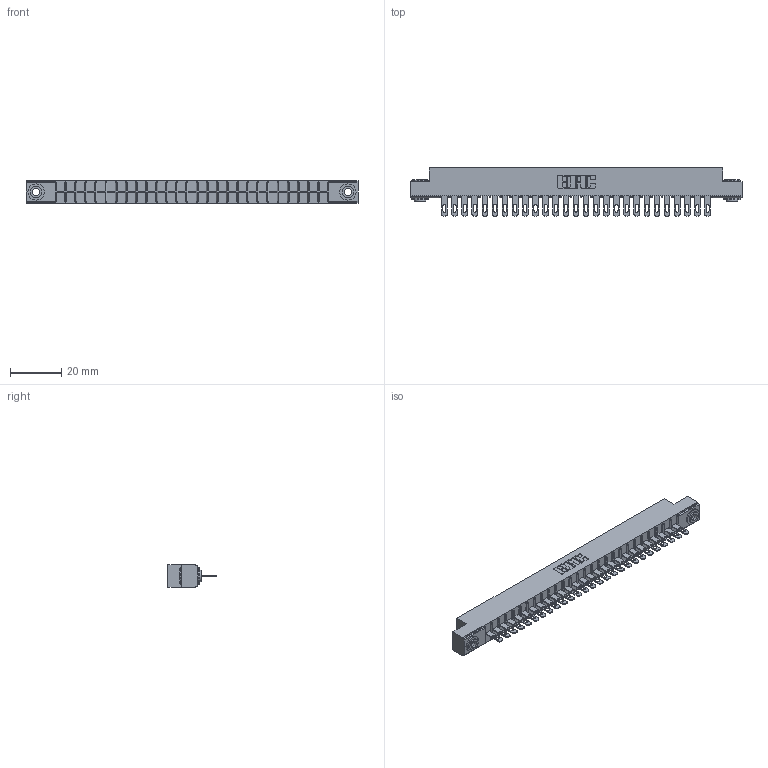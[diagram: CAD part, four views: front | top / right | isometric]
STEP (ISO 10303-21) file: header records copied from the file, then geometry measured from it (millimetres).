
FILE_DESCRIPTION (( 'STEP AP203' ), '1' );
FILE_NAME ('356-027-500-103.STEP', '2018-08-01T20:28:42', ( '' ), ( '' ), 'SwSTEP 2.0', 'SolidWorks 2016', '' );
FILE_SCHEMA (( 'CONFIG_CONTROL_DESIGN' ));
Length unit declared in the file: inch
Products named in the file (4): 356-027-500-103; 306 Part_.156 Dia; 306-290-001_100; 345-250-002_345-250-002-102
Assembly tree (30 placements, depth 2):
  356-027-500-103
    306 Part_.156 Dia
    306-290-001_100  x27
    345-250-002_345-250-002-102  x2
Bounding box: 130 x 18.87 x 8.71 mm (x, y, z)
Volume: 8997 mm3; surface area: 14151.2 mm2
Topology: 30 solids, 30 shells, 2220 faces, 6233 edges, 4006 vertices
Faces by surface type: plane 1442, cylinder 662, sphere 108, cone 8
Entity records: 28351 total; most frequent: CARTESIAN_POINT 4737, DIRECTION 4687, ORIENTED_EDGE 4686, EDGE_CURVE 2343, LINE 1815, VECTOR 1815, VERTEX_POINT 1486, AXIS2_PLACEMENT_3D 1436
